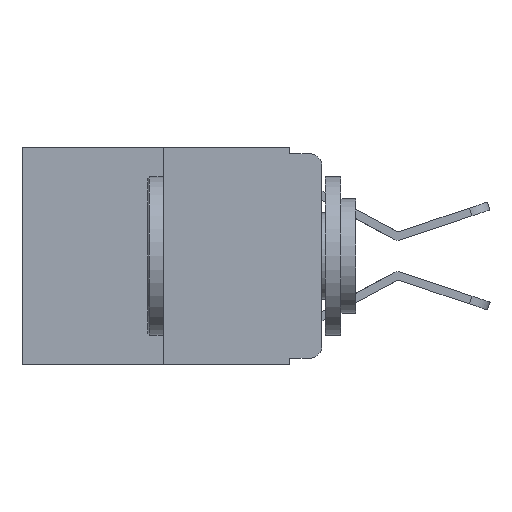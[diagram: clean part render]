
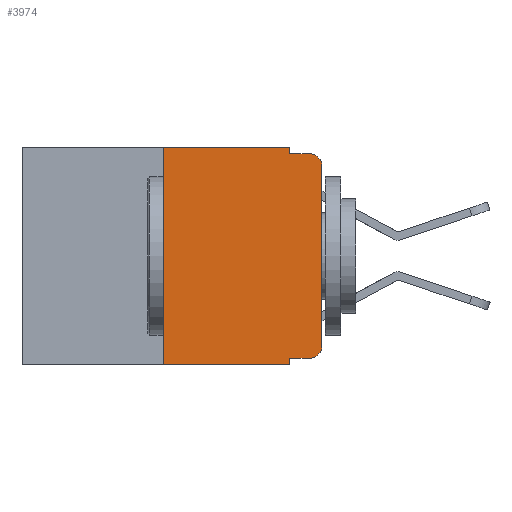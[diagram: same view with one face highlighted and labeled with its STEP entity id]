
A CAD part, left-side view. The second image highlights one B-rep face of the part: STEP entity #3974.
In plain terms, the highlighted planar face has unit normal (-1, 0, 0).
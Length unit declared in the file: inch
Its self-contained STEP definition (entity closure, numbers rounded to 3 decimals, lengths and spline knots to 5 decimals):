
#143 = CARTESIAN_POINT ( 'NONE',  ( 0., 0.473, -0.343 ) ) ;
#170 = LINE ( 'NONE', #9935, #4034 ) ;
#389 = VECTOR ( 'NONE', #2043, 39.37008 ) ;
#576 = CIRCLE ( 'NONE', #1192, 0.02 ) ;
#997 = DIRECTION ( 'NONE',  ( 0., 0., -1. ) ) ;
#1192 = AXIS2_PLACEMENT_3D ( 'NONE', #4509, #6921, #4702 ) ;
#1284 = VERTEX_POINT ( 'NONE', #13357 ) ;
#1749 = LINE ( 'NONE', #7801, #13063 ) ;
#1750 = VERTEX_POINT ( 'NONE', #1948 ) ;
#1948 = CARTESIAN_POINT ( 'NONE',  ( 0., 0., -0.03 ) ) ;
#2043 = DIRECTION ( 'NONE',  ( 0., -1., 0. ) ) ;
#2430 = CARTESIAN_POINT ( 'NONE',  ( 0., 0.02, -0.333 ) ) ;
#2891 = CARTESIAN_POINT ( 'NONE',  ( 0., 0.051, 0. ) ) ;
#2989 = VERTEX_POINT ( 'NONE', #5243 ) ;
#3330 = EDGE_CURVE ( 'NONE', #13624, #1284, #5394, .T. ) ;
#3359 = DIRECTION ( 'NONE',  ( 0., -1., 0. ) ) ;
#3402 = CARTESIAN_POINT ( 'NONE',  ( 0., 0.02, -0.313 ) ) ;
#3556 = VECTOR ( 'NONE', #997, 39.37008 ) ;
#3786 = LINE ( 'NONE', #4774, #5369 ) ;
#3845 = VECTOR ( 'NONE', #12364, 39.37008 ) ;
#3854 = CARTESIAN_POINT ( 'NONE',  ( 0., 0.25, -0.343 ) ) ;
#3974 = ADVANCED_FACE ( 'NONE', ( #10386 ), #11298, .F. ) ;
#4034 = VECTOR ( 'NONE', #12108, 39.37008 ) ;
#4095 = EDGE_CURVE ( 'NONE', #11746, #5757, #3786, .T. ) ;
#4137 = VERTEX_POINT ( 'NONE', #2891 ) ;
#4237 = LINE ( 'NONE', #7681, #389 ) ;
#4398 = AXIS2_PLACEMENT_3D ( 'NONE', #9103, #10439, #13814 ) ;
#4509 = CARTESIAN_POINT ( 'NONE',  ( 0., 0.02, -0.03 ) ) ;
#4533 = ORIENTED_EDGE ( 'NONE', *, *, #12700, .T. ) ;
#4702 = DIRECTION ( 'NONE',  ( 0., 0., -1. ) ) ;
#4774 = CARTESIAN_POINT ( 'NONE',  ( 0., 0.25, 0. ) ) ;
#5243 = CARTESIAN_POINT ( 'NONE',  ( 0., 0.051, -0.333 ) ) ;
#5369 = VECTOR ( 'NONE', #6952, 39.37008 ) ;
#5394 = CIRCLE ( 'NONE', #6827, 0.02 ) ;
#5736 = ORIENTED_EDGE ( 'NONE', *, *, #6711, .F. ) ;
#5757 = VERTEX_POINT ( 'NONE', #8902 ) ;
#5871 = EDGE_CURVE ( 'NONE', #1284, #1750, #12552, .T. ) ;
#6176 = LINE ( 'NONE', #14038, #3556 ) ;
#6214 = LINE ( 'NONE', #13238, #12619 ) ;
#6284 = EDGE_CURVE ( 'NONE', #5757, #4137, #170, .T. ) ;
#6433 = EDGE_CURVE ( 'NONE', #11746, #12801, #11828, .T. ) ;
#6711 = EDGE_CURVE ( 'NONE', #4137, #8776, #1749, .T. ) ;
#6827 = AXIS2_PLACEMENT_3D ( 'NONE', #3402, #11140, #11092 ) ;
#6921 = DIRECTION ( 'NONE',  ( -1., 0., 0. ) ) ;
#6952 = DIRECTION ( 'NONE',  ( 0., 0., 1. ) ) ;
#7681 = CARTESIAN_POINT ( 'NONE',  ( 0., 0.051, -0.01 ) ) ;
#7749 = ORIENTED_EDGE ( 'NONE', *, *, #6433, .T. ) ;
#7801 = CARTESIAN_POINT ( 'NONE',  ( 0., 0.051, 0. ) ) ;
#8458 = CARTESIAN_POINT ( 'NONE',  ( 0., 0.051, -0.01 ) ) ;
#8529 = CARTESIAN_POINT ( 'NONE',  ( 0., 0.02, -0.01 ) ) ;
#8776 = VERTEX_POINT ( 'NONE', #8458 ) ;
#8902 = CARTESIAN_POINT ( 'NONE',  ( 0., 0.25, 0. ) ) ;
#8992 = CARTESIAN_POINT ( 'NONE',  ( 0., 0.051, -0.343 ) ) ;
#9103 = CARTESIAN_POINT ( 'NONE',  ( 0., 0.473, 0. ) ) ;
#9296 = ORIENTED_EDGE ( 'NONE', *, *, #11366, .F. ) ;
#9813 = ORIENTED_EDGE ( 'NONE', *, *, #3330, .T. ) ;
#9935 = CARTESIAN_POINT ( 'NONE',  ( 0., 0.473, 0. ) ) ;
#10171 = EDGE_CURVE ( 'NONE', #2989, #13624, #6214, .T. ) ;
#10305 = ORIENTED_EDGE ( 'NONE', *, *, #6284, .F. ) ;
#10386 = FACE_OUTER_BOUND ( 'NONE', #10802, .T. ) ;
#10439 = DIRECTION ( 'NONE',  ( 1., 0., 0. ) ) ;
#10802 = EDGE_LOOP ( 'NONE', ( #14001, #4533, #12718, #5736, #10305, #13592, #7749, #9296, #11519, #9813 ) ) ;
#11092 = DIRECTION ( 'NONE',  ( 0., 0., -1. ) ) ;
#11140 = DIRECTION ( 'NONE',  ( -1., 0., 0. ) ) ;
#11298 = PLANE ( 'NONE',  #4398 ) ;
#11366 = EDGE_CURVE ( 'NONE', #2989, #12801, #6176, .T. ) ;
#11431 = CARTESIAN_POINT ( 'NONE',  ( 0., 0., 0. ) ) ;
#11519 = ORIENTED_EDGE ( 'NONE', *, *, #10171, .T. ) ;
#11746 = VERTEX_POINT ( 'NONE', #3854 ) ;
#11828 = LINE ( 'NONE', #143, #3845 ) ;
#12029 = VECTOR ( 'NONE', #12661, 39.37008 ) ;
#12108 = DIRECTION ( 'NONE',  ( 0., -1., 0. ) ) ;
#12364 = DIRECTION ( 'NONE',  ( 0., -1., 0. ) ) ;
#12552 = LINE ( 'NONE', #11431, #12029 ) ;
#12619 = VECTOR ( 'NONE', #3359, 39.37008 ) ;
#12661 = DIRECTION ( 'NONE',  ( 0., 0., 1. ) ) ;
#12700 = EDGE_CURVE ( 'NONE', #1750, #13866, #576, .T. ) ;
#12718 = ORIENTED_EDGE ( 'NONE', *, *, #13286, .F. ) ;
#12801 = VERTEX_POINT ( 'NONE', #8992 ) ;
#13063 = VECTOR ( 'NONE', #13369, 39.37008 ) ;
#13238 = CARTESIAN_POINT ( 'NONE',  ( 0., 0.051, -0.333 ) ) ;
#13286 = EDGE_CURVE ( 'NONE', #8776, #13866, #4237, .T. ) ;
#13357 = CARTESIAN_POINT ( 'NONE',  ( 0., 0., -0.313 ) ) ;
#13369 = DIRECTION ( 'NONE',  ( 0., 0., -1. ) ) ;
#13592 = ORIENTED_EDGE ( 'NONE', *, *, #4095, .F. ) ;
#13624 = VERTEX_POINT ( 'NONE', #2430 ) ;
#13814 = DIRECTION ( 'NONE',  ( 0., 0., -1. ) ) ;
#13866 = VERTEX_POINT ( 'NONE', #8529 ) ;
#14001 = ORIENTED_EDGE ( 'NONE', *, *, #5871, .T. ) ;
#14038 = CARTESIAN_POINT ( 'NONE',  ( 0., 0.051, 0. ) ) ;
